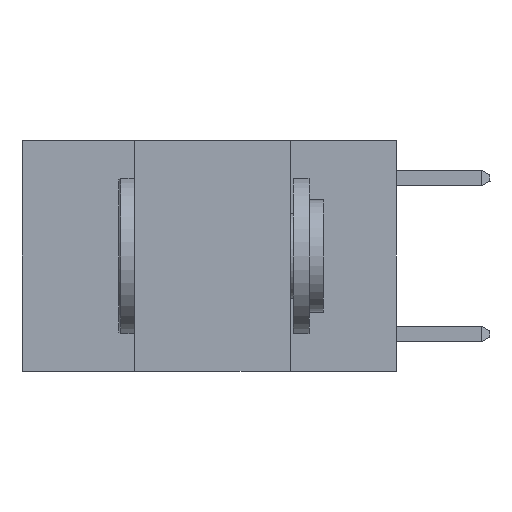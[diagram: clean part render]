
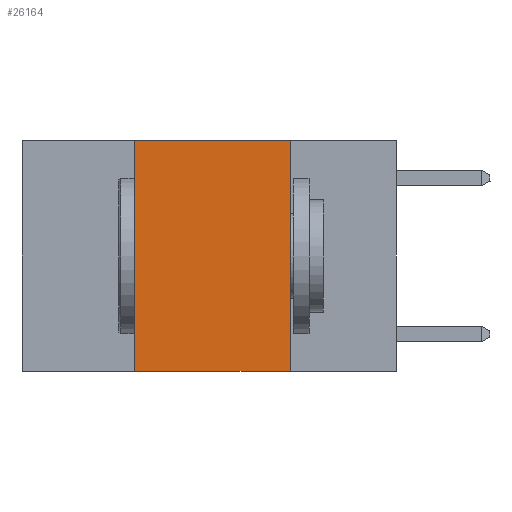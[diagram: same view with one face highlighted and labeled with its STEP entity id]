
A CAD part, left-side view. The second image highlights one B-rep face of the part: STEP entity #26164.
In plain terms, the highlighted planar face has unit normal (-1, 0, 0).
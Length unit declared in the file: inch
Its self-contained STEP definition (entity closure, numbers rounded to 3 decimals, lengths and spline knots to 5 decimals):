
#267 = CARTESIAN_POINT ( 'NONE',  ( 0., 0.42, 0. ) ) ;
#315 = VECTOR ( 'NONE', #18616, 39.37008 ) ;
#347 = EDGE_CURVE ( 'NONE', #15836, #5813, #19622, .T. ) ;
#397 = CARTESIAN_POINT ( 'NONE',  ( 0., 0.42, 0. ) ) ;
#1101 = LINE ( 'NONE', #22238, #25728 ) ;
#1188 = VECTOR ( 'NONE', #13838, 39.37008 ) ;
#1343 = DIRECTION ( 'NONE',  ( 0., -1., 0. ) ) ;
#3392 = ORIENTED_EDGE ( 'NONE', *, *, #4334, .F. ) ;
#3631 = ORIENTED_EDGE ( 'NONE', *, *, #27637, .F. ) ;
#3789 = ORIENTED_EDGE ( 'NONE', *, *, #347, .F. ) ;
#4210 = ORIENTED_EDGE ( 'NONE', *, *, #26538, .T. ) ;
#4334 = EDGE_CURVE ( 'NONE', #29190, #24625, #1101, .T. ) ;
#4727 = FACE_OUTER_BOUND ( 'NONE', #18285, .T. ) ;
#4928 = DIRECTION ( 'NONE',  ( 0., 0., -1. ) ) ;
#5813 = VERTEX_POINT ( 'NONE', #397 ) ;
#10565 = DIRECTION ( 'NONE',  ( 0., 0., -1. ) ) ;
#11397 = CARTESIAN_POINT ( 'NONE',  ( 0., 0.6, 0. ) ) ;
#13838 = DIRECTION ( 'NONE',  ( 0., -1., 0. ) ) ;
#14657 = PLANE ( 'NONE',  #16158 ) ;
#14988 = LINE ( 'NONE', #11397, #1188 ) ;
#15836 = VERTEX_POINT ( 'NONE', #22897 ) ;
#16158 = AXIS2_PLACEMENT_3D ( 'NONE', #17022, #19305, #4928 ) ;
#17022 = CARTESIAN_POINT ( 'NONE',  ( 0., 0.6, 0. ) ) ;
#18285 = EDGE_LOOP ( 'NONE', ( #3392, #3631, #3789, #4210 ) ) ;
#18286 = CARTESIAN_POINT ( 'NONE',  ( 0., 0.17, -0.37 ) ) ;
#18616 = DIRECTION ( 'NONE',  ( 0., 0., 1. ) ) ;
#19305 = DIRECTION ( 'NONE',  ( 1., 0., 0. ) ) ;
#19622 = LINE ( 'NONE', #267, #315 ) ;
#19706 = LINE ( 'NONE', #22811, #29855 ) ;
#22238 = CARTESIAN_POINT ( 'NONE',  ( 0., 0.17, 0. ) ) ;
#22811 = CARTESIAN_POINT ( 'NONE',  ( 0., 0.6, -0.37 ) ) ;
#22897 = CARTESIAN_POINT ( 'NONE',  ( 0., 0.42, -0.37 ) ) ;
#24625 = VERTEX_POINT ( 'NONE', #18286 ) ;
#25728 = VECTOR ( 'NONE', #10565, 39.37008 ) ;
#26164 = ADVANCED_FACE ( 'NONE', ( #4727 ), #14657, .F. ) ;
#26538 = EDGE_CURVE ( 'NONE', #15836, #24625, #19706, .T. ) ;
#27637 = EDGE_CURVE ( 'NONE', #5813, #29190, #14988, .T. ) ;
#29190 = VERTEX_POINT ( 'NONE', #30461 ) ;
#29855 = VECTOR ( 'NONE', #1343, 39.37008 ) ;
#30461 = CARTESIAN_POINT ( 'NONE',  ( 0., 0.17, 0. ) ) ;
